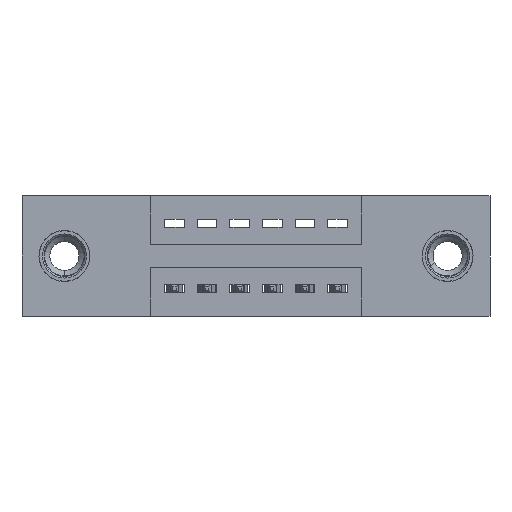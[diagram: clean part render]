
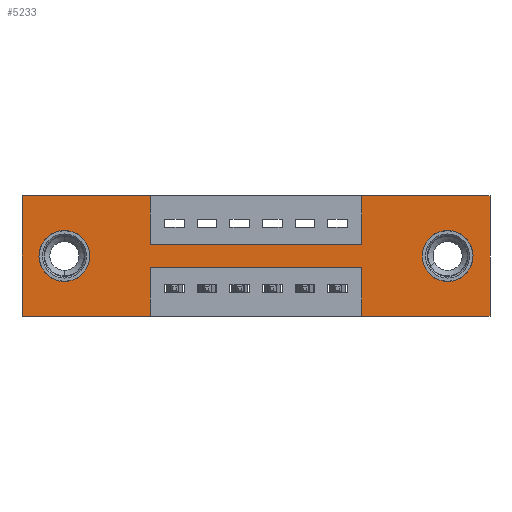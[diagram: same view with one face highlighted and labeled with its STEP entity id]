
A CAD part, front view. The second image highlights one B-rep face of the part: STEP entity #5233.
In plain terms, the highlighted planar face has unit normal (0, -1, 0).
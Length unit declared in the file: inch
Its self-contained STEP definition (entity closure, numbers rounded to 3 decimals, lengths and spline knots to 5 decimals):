
#44 = LINE ( 'NONE', #4613, #1907 ) ;
#64 = VERTEX_POINT ( 'NONE', #4017 ) ;
#123 = DIRECTION ( 'NONE',  ( 0., 0., 1. ) ) ;
#221 = VERTEX_POINT ( 'NONE', #7693 ) ;
#288 = VERTEX_POINT ( 'NONE', #2097 ) ;
#408 = ORIENTED_EDGE ( 'NONE', *, *, #3686, .F. ) ;
#521 = ORIENTED_EDGE ( 'NONE', *, *, #6227, .F. ) ;
#1032 = LINE ( 'NONE', #3278, #9496 ) ;
#1055 = FACE_BOUND ( 'NONE', #1736, .T. ) ;
#1289 = LINE ( 'NONE', #7381, #8587 ) ;
#1568 = DIRECTION ( 'NONE',  ( -1., 0., 0. ) ) ;
#1575 = EDGE_CURVE ( 'NONE', #64, #9234, #10172, .T. ) ;
#1610 = CARTESIAN_POINT ( 'NONE',  ( 0., 0., -0.37 ) ) ;
#1707 = CARTESIAN_POINT ( 'NONE',  ( 0.13, 0., -0.185 ) ) ;
#1712 = ORIENTED_EDGE ( 'NONE', *, *, #8720, .F. ) ;
#1736 = EDGE_LOOP ( 'NONE', ( #9301, #10207 ) ) ;
#1907 = VECTOR ( 'NONE', #9582, 39.37008 ) ;
#1949 = VERTEX_POINT ( 'NONE', #4852 ) ;
#1977 = LINE ( 'NONE', #2789, #5789 ) ;
#2009 = CARTESIAN_POINT ( 'NONE',  ( 1.0425, 0., 0. ) ) ;
#2097 = CARTESIAN_POINT ( 'NONE',  ( 1.0425, 0., -0.15 ) ) ;
#2101 = VERTEX_POINT ( 'NONE', #8150 ) ;
#2130 = EDGE_CURVE ( 'NONE', #3141, #6463, #4421, .T. ) ;
#2145 = ORIENTED_EDGE ( 'NONE', *, *, #3505, .F. ) ;
#2307 = CIRCLE ( 'NONE', #8986, 0.078 ) ;
#2337 = CARTESIAN_POINT ( 'NONE',  ( 0., 0., -0.37 ) ) ;
#2340 = EDGE_CURVE ( 'NONE', #3727, #3141, #1977, .T. ) ;
#2396 = LINE ( 'NONE', #6606, #4561 ) ;
#2408 = CARTESIAN_POINT ( 'NONE',  ( 0.3925, 0., 0. ) ) ;
#2494 = LINE ( 'NONE', #9483, #2731 ) ;
#2672 = AXIS2_PLACEMENT_3D ( 'NONE', #3366, #4195, #123 ) ;
#2731 = VECTOR ( 'NONE', #8676, 39.37008 ) ;
#2789 = CARTESIAN_POINT ( 'NONE',  ( 0., 0., 0. ) ) ;
#2796 = VECTOR ( 'NONE', #5048, 39.37008 ) ;
#2919 = VERTEX_POINT ( 'NONE', #5634 ) ;
#3063 = CARTESIAN_POINT ( 'NONE',  ( 0.3925, 0., -0.22 ) ) ;
#3080 = LINE ( 'NONE', #5267, #9361 ) ;
#3132 = CARTESIAN_POINT ( 'NONE',  ( 1.305, 0., -0.185 ) ) ;
#3141 = VERTEX_POINT ( 'NONE', #4767 ) ;
#3278 = CARTESIAN_POINT ( 'NONE',  ( 0., 0., 0. ) ) ;
#3322 = VERTEX_POINT ( 'NONE', #7724 ) ;
#3366 = CARTESIAN_POINT ( 'NONE',  ( 0.13, 0., -0.185 ) ) ;
#3388 = ORIENTED_EDGE ( 'NONE', *, *, #3477, .F. ) ;
#3453 = ORIENTED_EDGE ( 'NONE', *, *, #8672, .F. ) ;
#3477 = EDGE_CURVE ( 'NONE', #8598, #2919, #2494, .T. ) ;
#3505 = EDGE_CURVE ( 'NONE', #288, #3322, #5297, .T. ) ;
#3686 = EDGE_CURVE ( 'NONE', #2919, #9590, #6168, .T. ) ;
#3727 = VERTEX_POINT ( 'NONE', #1610 ) ;
#3867 = DIRECTION ( 'NONE',  ( 0., 0., -1. ) ) ;
#3985 = ORIENTED_EDGE ( 'NONE', *, *, #9064, .F. ) ;
#4010 = ORIENTED_EDGE ( 'NONE', *, *, #9207, .F. ) ;
#4017 = CARTESIAN_POINT ( 'NONE',  ( 0.13, 0., -0.107 ) ) ;
#4126 = CIRCLE ( 'NONE', #5356, 0.078 ) ;
#4185 = CARTESIAN_POINT ( 'NONE',  ( 1.0425, 0., -0.37 ) ) ;
#4195 = DIRECTION ( 'NONE',  ( 0., 1., 0. ) ) ;
#4421 = LINE ( 'NONE', #5454, #4950 ) ;
#4561 = VECTOR ( 'NONE', #8054, 39.37008 ) ;
#4595 = LINE ( 'NONE', #4185, #2796 ) ;
#4613 = CARTESIAN_POINT ( 'NONE',  ( 0.3925, 0., -0.15 ) ) ;
#4632 = ORIENTED_EDGE ( 'NONE', *, *, #6508, .T. ) ;
#4767 = CARTESIAN_POINT ( 'NONE',  ( 0., 0., 0. ) ) ;
#4786 = DIRECTION ( 'NONE',  ( 1., 0., 0. ) ) ;
#4790 = VECTOR ( 'NONE', #9401, 39.37008 ) ;
#4852 = CARTESIAN_POINT ( 'NONE',  ( 1.305, 0., -0.107 ) ) ;
#4881 = ORIENTED_EDGE ( 'NONE', *, *, #2340, .F. ) ;
#4892 = EDGE_LOOP ( 'NONE', ( #1712, #3453, #10109, #408, #3388, #521, #2145, #4010, #5221, #10133, #4881, #3985 ) ) ;
#4950 = VECTOR ( 'NONE', #4786, 39.37008 ) ;
#5001 = DIRECTION ( 'NONE',  ( 1., 0., 0. ) ) ;
#5048 = DIRECTION ( 'NONE',  ( 0., 0., 1. ) ) ;
#5221 = ORIENTED_EDGE ( 'NONE', *, *, #7404, .F. ) ;
#5233 = ADVANCED_FACE ( 'NONE', ( #1055, #9249, #7034 ), #5329, .T. ) ;
#5267 = CARTESIAN_POINT ( 'NONE',  ( 0., 0., -0.37 ) ) ;
#5297 = LINE ( 'NONE', #2009, #4790 ) ;
#5329 = PLANE ( 'NONE',  #5582 ) ;
#5356 = AXIS2_PLACEMENT_3D ( 'NONE', #3132, #9773, #9710 ) ;
#5359 = CIRCLE ( 'NONE', #2672, 0.078 ) ;
#5454 = CARTESIAN_POINT ( 'NONE',  ( 0., 0., 0. ) ) ;
#5530 = DIRECTION ( 'NONE',  ( -1., 0., 0. ) ) ;
#5555 = CARTESIAN_POINT ( 'NONE',  ( 1.305, 0., -0.185 ) ) ;
#5582 = AXIS2_PLACEMENT_3D ( 'NONE', #6994, #10348, #7030 ) ;
#5592 = EDGE_CURVE ( 'NONE', #1949, #2101, #2307, .T. ) ;
#5634 = CARTESIAN_POINT ( 'NONE',  ( 1.435, 0., -0.37 ) ) ;
#5789 = VECTOR ( 'NONE', #9329, 39.37008 ) ;
#5798 = DIRECTION ( 'NONE',  ( 0., 0., 1. ) ) ;
#6046 = DIRECTION ( 'NONE',  ( -1., 0., 0. ) ) ;
#6143 = EDGE_CURVE ( 'NONE', #9590, #10192, #4595, .T. ) ;
#6168 = LINE ( 'NONE', #2337, #7315 ) ;
#6204 = ORIENTED_EDGE ( 'NONE', *, *, #1575, .T. ) ;
#6227 = EDGE_CURVE ( 'NONE', #3322, #8598, #1032, .T. ) ;
#6463 = VERTEX_POINT ( 'NONE', #2408 ) ;
#6508 = EDGE_CURVE ( 'NONE', #9234, #64, #5359, .T. ) ;
#6606 = CARTESIAN_POINT ( 'NONE',  ( 0.3925, 0., 0. ) ) ;
#6994 = CARTESIAN_POINT ( 'NONE',  ( 0., 0., -0.37 ) ) ;
#7030 = DIRECTION ( 'NONE',  ( 0., 0., -1. ) ) ;
#7034 = FACE_OUTER_BOUND ( 'NONE', #4892, .T. ) ;
#7277 = LINE ( 'NONE', #9793, #8847 ) ;
#7315 = VECTOR ( 'NONE', #5530, 39.37008 ) ;
#7381 = CARTESIAN_POINT ( 'NONE',  ( 0.3925, 0., -0.37 ) ) ;
#7404 = EDGE_CURVE ( 'NONE', #6463, #7504, #2396, .T. ) ;
#7504 = VERTEX_POINT ( 'NONE', #7921 ) ;
#7549 = CARTESIAN_POINT ( 'NONE',  ( 0.13, 0., -0.263 ) ) ;
#7693 = CARTESIAN_POINT ( 'NONE',  ( 0.3925, 0., -0.37 ) ) ;
#7711 = CARTESIAN_POINT ( 'NONE',  ( 1.0425, 0., -0.37 ) ) ;
#7724 = CARTESIAN_POINT ( 'NONE',  ( 1.0425, 0., 0. ) ) ;
#7886 = VERTEX_POINT ( 'NONE', #3063 ) ;
#7921 = CARTESIAN_POINT ( 'NONE',  ( 0.3925, 0., -0.15 ) ) ;
#7951 = EDGE_CURVE ( 'NONE', #2101, #1949, #4126, .T. ) ;
#8054 = DIRECTION ( 'NONE',  ( 0., 0., -1. ) ) ;
#8150 = CARTESIAN_POINT ( 'NONE',  ( 1.305, 0., -0.263 ) ) ;
#8264 = DIRECTION ( 'NONE',  ( 0., 1., 0. ) ) ;
#8331 = DIRECTION ( 'NONE',  ( 0., 0., -1. ) ) ;
#8587 = VECTOR ( 'NONE', #8331, 39.37008 ) ;
#8598 = VERTEX_POINT ( 'NONE', #9097 ) ;
#8672 = EDGE_CURVE ( 'NONE', #10192, #7886, #7277, .T. ) ;
#8676 = DIRECTION ( 'NONE',  ( 0., 0., -1. ) ) ;
#8720 = EDGE_CURVE ( 'NONE', #7886, #221, #1289, .T. ) ;
#8847 = VECTOR ( 'NONE', #1568, 39.37008 ) ;
#8915 = DIRECTION ( 'NONE',  ( 0., 1., 0. ) ) ;
#8986 = AXIS2_PLACEMENT_3D ( 'NONE', #5555, #8915, #3867 ) ;
#9064 = EDGE_CURVE ( 'NONE', #221, #3727, #3080, .T. ) ;
#9097 = CARTESIAN_POINT ( 'NONE',  ( 1.435, 0., 0. ) ) ;
#9207 = EDGE_CURVE ( 'NONE', #7504, #288, #44, .T. ) ;
#9234 = VERTEX_POINT ( 'NONE', #7549 ) ;
#9249 = FACE_BOUND ( 'NONE', #9965, .T. ) ;
#9301 = ORIENTED_EDGE ( 'NONE', *, *, #5592, .T. ) ;
#9329 = DIRECTION ( 'NONE',  ( 0., 0., 1. ) ) ;
#9361 = VECTOR ( 'NONE', #6046, 39.37008 ) ;
#9365 = AXIS2_PLACEMENT_3D ( 'NONE', #1707, #8264, #5798 ) ;
#9401 = DIRECTION ( 'NONE',  ( 0., 0., 1. ) ) ;
#9450 = CARTESIAN_POINT ( 'NONE',  ( 1.0425, 0., -0.22 ) ) ;
#9483 = CARTESIAN_POINT ( 'NONE',  ( 1.435, 0., 0. ) ) ;
#9496 = VECTOR ( 'NONE', #5001, 39.37008 ) ;
#9582 = DIRECTION ( 'NONE',  ( 1., 0., 0. ) ) ;
#9590 = VERTEX_POINT ( 'NONE', #7711 ) ;
#9710 = DIRECTION ( 'NONE',  ( 0., 0., -1. ) ) ;
#9773 = DIRECTION ( 'NONE',  ( 0., 1., 0. ) ) ;
#9793 = CARTESIAN_POINT ( 'NONE',  ( 0.3925, 0., -0.22 ) ) ;
#9965 = EDGE_LOOP ( 'NONE', ( #6204, #4632 ) ) ;
#10109 = ORIENTED_EDGE ( 'NONE', *, *, #6143, .F. ) ;
#10133 = ORIENTED_EDGE ( 'NONE', *, *, #2130, .F. ) ;
#10172 = CIRCLE ( 'NONE', #9365, 0.078 ) ;
#10192 = VERTEX_POINT ( 'NONE', #9450 ) ;
#10207 = ORIENTED_EDGE ( 'NONE', *, *, #7951, .T. ) ;
#10348 = DIRECTION ( 'NONE',  ( 0., -1., 0. ) ) ;
